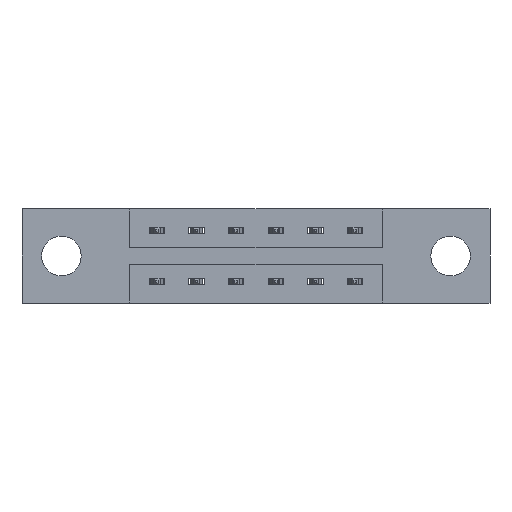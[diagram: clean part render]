
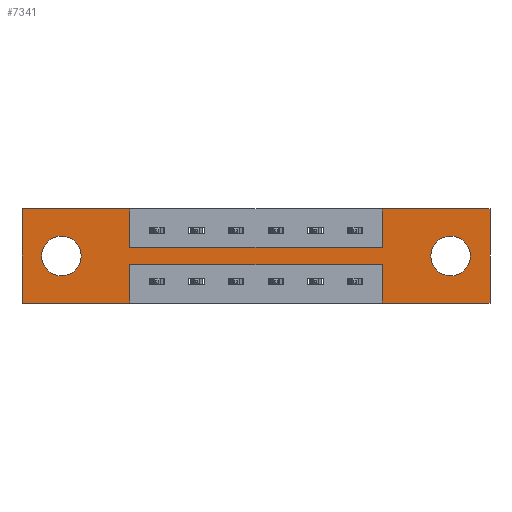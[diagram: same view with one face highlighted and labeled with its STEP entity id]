
A CAD part, front view. The second image highlights one B-rep face of the part: STEP entity #7341.
In plain terms, the highlighted planar face has unit normal (0, -1, 0).
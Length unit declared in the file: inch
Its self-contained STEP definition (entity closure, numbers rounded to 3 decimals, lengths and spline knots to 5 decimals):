
#4 = ORIENTED_EDGE ( 'NONE', *, *, #1456, .F. ) ;
#34 = EDGE_CURVE ( 'NONE', #5607, #1265, #5023, .T. ) ;
#56 = CARTESIAN_POINT ( 'NONE',  ( 1.417, 0., 0. ) ) ;
#67 = ORIENTED_EDGE ( 'NONE', *, *, #6719, .F. ) ;
#300 = CARTESIAN_POINT ( 'NONE',  ( 1.687, 0., -0.107 ) ) ;
#382 = DIRECTION ( 'NONE',  ( 0., 0., -1. ) ) ;
#575 = EDGE_CURVE ( 'NONE', #8751, #5078, #6491, .T. ) ;
#600 = ORIENTED_EDGE ( 'NONE', *, *, #6470, .T. ) ;
#611 = ORIENTED_EDGE ( 'NONE', *, *, #5725, .F. ) ;
#634 = CARTESIAN_POINT ( 'NONE',  ( 0., 0., 0. ) ) ;
#709 = DIRECTION ( 'NONE',  ( 0., 0., -1. ) ) ;
#734 = CARTESIAN_POINT ( 'NONE',  ( 0., 0., 0. ) ) ;
#821 = FACE_BOUND ( 'NONE', #7486, .T. ) ;
#909 = CARTESIAN_POINT ( 'NONE',  ( 1.687, 0., -0.185 ) ) ;
#942 = CARTESIAN_POINT ( 'NONE',  ( 0.155, 0., -0.185 ) ) ;
#953 = LINE ( 'NONE', #7181, #4313 ) ;
#996 = CARTESIAN_POINT ( 'NONE',  ( 1.417, 0., -0.37 ) ) ;
#1100 = VECTOR ( 'NONE', #5349, 39.37008 ) ;
#1161 = EDGE_CURVE ( 'NONE', #2240, #7572, #8088, .T. ) ;
#1212 = EDGE_LOOP ( 'NONE', ( #1859, #6642 ) ) ;
#1225 = CARTESIAN_POINT ( 'NONE',  ( 0.425, 0., 0. ) ) ;
#1242 = EDGE_CURVE ( 'NONE', #2482, #1630, #5373, .T. ) ;
#1265 = VERTEX_POINT ( 'NONE', #8293 ) ;
#1300 = DIRECTION ( 'NONE',  ( 0., 0., 1. ) ) ;
#1305 = ORIENTED_EDGE ( 'NONE', *, *, #2187, .F. ) ;
#1306 = AXIS2_PLACEMENT_3D ( 'NONE', #942, #3798, #6566 ) ;
#1384 = VECTOR ( 'NONE', #1865, 39.37008 ) ;
#1415 = CIRCLE ( 'NONE', #3568, 0.078 ) ;
#1436 = CARTESIAN_POINT ( 'NONE',  ( 0.425, 0., -0.37 ) ) ;
#1456 = EDGE_CURVE ( 'NONE', #4852, #4512, #7167, .T. ) ;
#1540 = VECTOR ( 'NONE', #2838, 39.37008 ) ;
#1564 = CARTESIAN_POINT ( 'NONE',  ( 0.425, 0., -0.22 ) ) ;
#1566 = VECTOR ( 'NONE', #6649, 39.37008 ) ;
#1594 = FACE_BOUND ( 'NONE', #1212, .T. ) ;
#1630 = VERTEX_POINT ( 'NONE', #6362 ) ;
#1781 = CARTESIAN_POINT ( 'NONE',  ( 0., 0., -0.37 ) ) ;
#1807 = CARTESIAN_POINT ( 'NONE',  ( 1.842, 0., 0. ) ) ;
#1859 = ORIENTED_EDGE ( 'NONE', *, *, #4335, .T. ) ;
#1865 = DIRECTION ( 'NONE',  ( 0., 0., -1. ) ) ;
#1927 = LINE ( 'NONE', #734, #3393 ) ;
#1932 = ORIENTED_EDGE ( 'NONE', *, *, #1242, .T. ) ;
#2113 = CARTESIAN_POINT ( 'NONE',  ( 1.687, 0., -0.185 ) ) ;
#2187 = EDGE_CURVE ( 'NONE', #8807, #4852, #1927, .T. ) ;
#2240 = VERTEX_POINT ( 'NONE', #4176 ) ;
#2294 = ORIENTED_EDGE ( 'NONE', *, *, #3279, .F. ) ;
#2417 = DIRECTION ( 'NONE',  ( 0., 0., 1. ) ) ;
#2460 = CARTESIAN_POINT ( 'NONE',  ( 0.425, 0., -0.15 ) ) ;
#2482 = VERTEX_POINT ( 'NONE', #300 ) ;
#2629 = ORIENTED_EDGE ( 'NONE', *, *, #34, .F. ) ;
#2795 = ORIENTED_EDGE ( 'NONE', *, *, #8792, .F. ) ;
#2813 = LINE ( 'NONE', #1807, #4630 ) ;
#2838 = DIRECTION ( 'NONE',  ( 1., 0., 0. ) ) ;
#3050 = CARTESIAN_POINT ( 'NONE',  ( 0., 0., -0.37 ) ) ;
#3073 = DIRECTION ( 'NONE',  ( 0., 0., -1. ) ) ;
#3133 = VECTOR ( 'NONE', #6832, 39.37008 ) ;
#3273 = CARTESIAN_POINT ( 'NONE',  ( 1.842, 0., -0.37 ) ) ;
#3279 = EDGE_CURVE ( 'NONE', #4311, #4073, #8253, .T. ) ;
#3346 = VECTOR ( 'NONE', #7324, 39.37008 ) ;
#3393 = VECTOR ( 'NONE', #6127, 39.37008 ) ;
#3468 = EDGE_LOOP ( 'NONE', ( #5367, #5818, #611, #4990, #2795, #2629, #7786, #6998, #4, #1305, #67, #2294 ) ) ;
#3503 = CARTESIAN_POINT ( 'NONE',  ( 0., 0., 0. ) ) ;
#3530 = LINE ( 'NONE', #7760, #1384 ) ;
#3568 = AXIS2_PLACEMENT_3D ( 'NONE', #7295, #3621, #8664 ) ;
#3621 = DIRECTION ( 'NONE',  ( 0., 1., 0. ) ) ;
#3798 = DIRECTION ( 'NONE',  ( 0., 1., 0. ) ) ;
#4073 = VERTEX_POINT ( 'NONE', #3050 ) ;
#4176 = CARTESIAN_POINT ( 'NONE',  ( 0.155, 0., -0.263 ) ) ;
#4306 = FACE_OUTER_BOUND ( 'NONE', #3468, .T. ) ;
#4311 = VERTEX_POINT ( 'NONE', #1436 ) ;
#4313 = VECTOR ( 'NONE', #5015, 39.37008 ) ;
#4335 = EDGE_CURVE ( 'NONE', #7572, #2240, #1415, .T. ) ;
#4389 = VECTOR ( 'NONE', #1300, 39.37008 ) ;
#4512 = VERTEX_POINT ( 'NONE', #7925 ) ;
#4612 = EDGE_CURVE ( 'NONE', #4512, #4749, #6380, .T. ) ;
#4630 = VECTOR ( 'NONE', #8317, 39.37008 ) ;
#4652 = AXIS2_PLACEMENT_3D ( 'NONE', #909, #5941, #3073 ) ;
#4705 = EDGE_CURVE ( 'NONE', #4803, #5691, #7311, .T. ) ;
#4749 = VERTEX_POINT ( 'NONE', #8959 ) ;
#4803 = VERTEX_POINT ( 'NONE', #3273 ) ;
#4852 = VERTEX_POINT ( 'NONE', #7642 ) ;
#4990 = ORIENTED_EDGE ( 'NONE', *, *, #4705, .F. ) ;
#4993 = VECTOR ( 'NONE', #2417, 39.37008 ) ;
#5015 = DIRECTION ( 'NONE',  ( 0., 0., 1. ) ) ;
#5023 = LINE ( 'NONE', #3503, #1540 ) ;
#5078 = VERTEX_POINT ( 'NONE', #7318 ) ;
#5122 = CARTESIAN_POINT ( 'NONE',  ( 0.155, 0., -0.107 ) ) ;
#5251 = VECTOR ( 'NONE', #6923, 39.37008 ) ;
#5276 = CARTESIAN_POINT ( 'NONE',  ( 1.417, 0., -0.37 ) ) ;
#5286 = CARTESIAN_POINT ( 'NONE',  ( 0., 0., -0.37 ) ) ;
#5349 = DIRECTION ( 'NONE',  ( 1., 0., 0. ) ) ;
#5367 = ORIENTED_EDGE ( 'NONE', *, *, #6321, .F. ) ;
#5373 = CIRCLE ( 'NONE', #4652, 0.078 ) ;
#5607 = VERTEX_POINT ( 'NONE', #56 ) ;
#5691 = VERTEX_POINT ( 'NONE', #996 ) ;
#5725 = EDGE_CURVE ( 'NONE', #5691, #8751, #8531, .T. ) ;
#5818 = ORIENTED_EDGE ( 'NONE', *, *, #575, .F. ) ;
#5941 = DIRECTION ( 'NONE',  ( 0., 1., 0. ) ) ;
#6127 = DIRECTION ( 'NONE',  ( 1., 0., 0. ) ) ;
#6321 = EDGE_CURVE ( 'NONE', #5078, #4311, #3530, .T. ) ;
#6362 = CARTESIAN_POINT ( 'NONE',  ( 1.687, 0., -0.263 ) ) ;
#6380 = LINE ( 'NONE', #2460, #1100 ) ;
#6470 = EDGE_CURVE ( 'NONE', #1630, #2482, #7145, .T. ) ;
#6491 = LINE ( 'NONE', #1564, #3346 ) ;
#6566 = DIRECTION ( 'NONE',  ( 0., 0., 1. ) ) ;
#6642 = ORIENTED_EDGE ( 'NONE', *, *, #1161, .T. ) ;
#6649 = DIRECTION ( 'NONE',  ( -1., 0., 0. ) ) ;
#6719 = EDGE_CURVE ( 'NONE', #4073, #8807, #953, .T. ) ;
#6742 = CARTESIAN_POINT ( 'NONE',  ( 0., 0., -0.37 ) ) ;
#6832 = DIRECTION ( 'NONE',  ( -1., 0., 0. ) ) ;
#6923 = DIRECTION ( 'NONE',  ( 0., 0., -1. ) ) ;
#6924 = PLANE ( 'NONE',  #8825 ) ;
#6993 = LINE ( 'NONE', #9257, #4389 ) ;
#6998 = ORIENTED_EDGE ( 'NONE', *, *, #4612, .F. ) ;
#7145 = CIRCLE ( 'NONE', #8500, 0.078 ) ;
#7167 = LINE ( 'NONE', #1225, #5251 ) ;
#7181 = CARTESIAN_POINT ( 'NONE',  ( 0., 0., 0. ) ) ;
#7295 = CARTESIAN_POINT ( 'NONE',  ( 0.155, 0., -0.185 ) ) ;
#7311 = LINE ( 'NONE', #5286, #3133 ) ;
#7318 = CARTESIAN_POINT ( 'NONE',  ( 0.425, 0., -0.22 ) ) ;
#7324 = DIRECTION ( 'NONE',  ( -1., 0., 0. ) ) ;
#7341 = ADVANCED_FACE ( 'NONE', ( #821, #1594, #4306 ), #6924, .T. ) ;
#7486 = EDGE_LOOP ( 'NONE', ( #1932, #600 ) ) ;
#7570 = DIRECTION ( 'NONE',  ( 0., -1., 0. ) ) ;
#7572 = VERTEX_POINT ( 'NONE', #5122 ) ;
#7642 = CARTESIAN_POINT ( 'NONE',  ( 0.425, 0., 0. ) ) ;
#7760 = CARTESIAN_POINT ( 'NONE',  ( 0.425, 0., -0.37 ) ) ;
#7786 = ORIENTED_EDGE ( 'NONE', *, *, #9100, .F. ) ;
#7925 = CARTESIAN_POINT ( 'NONE',  ( 0.425, 0., -0.15 ) ) ;
#8088 = CIRCLE ( 'NONE', #1306, 0.078 ) ;
#8164 = CARTESIAN_POINT ( 'NONE',  ( 1.417, 0., -0.22 ) ) ;
#8253 = LINE ( 'NONE', #6742, #1566 ) ;
#8293 = CARTESIAN_POINT ( 'NONE',  ( 1.842, 0., 0. ) ) ;
#8317 = DIRECTION ( 'NONE',  ( 0., 0., -1. ) ) ;
#8500 = AXIS2_PLACEMENT_3D ( 'NONE', #2113, #8636, #709 ) ;
#8531 = LINE ( 'NONE', #5276, #4993 ) ;
#8636 = DIRECTION ( 'NONE',  ( 0., 1., 0. ) ) ;
#8664 = DIRECTION ( 'NONE',  ( 0., 0., 1. ) ) ;
#8751 = VERTEX_POINT ( 'NONE', #8164 ) ;
#8792 = EDGE_CURVE ( 'NONE', #1265, #4803, #2813, .T. ) ;
#8807 = VERTEX_POINT ( 'NONE', #634 ) ;
#8825 = AXIS2_PLACEMENT_3D ( 'NONE', #1781, #7570, #382 ) ;
#8959 = CARTESIAN_POINT ( 'NONE',  ( 1.417, 0., -0.15 ) ) ;
#9100 = EDGE_CURVE ( 'NONE', #4749, #5607, #6993, .T. ) ;
#9257 = CARTESIAN_POINT ( 'NONE',  ( 1.417, 0., 0. ) ) ;
